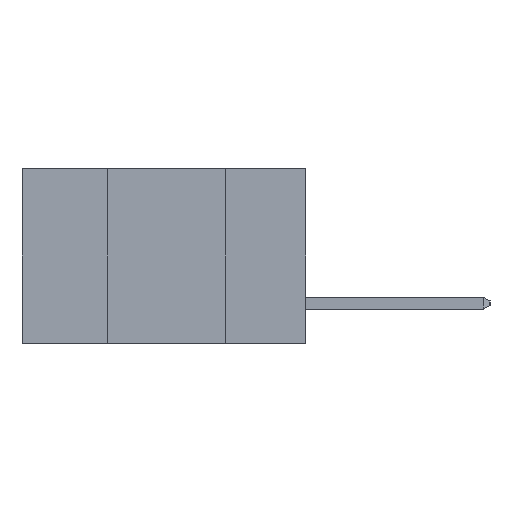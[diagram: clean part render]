
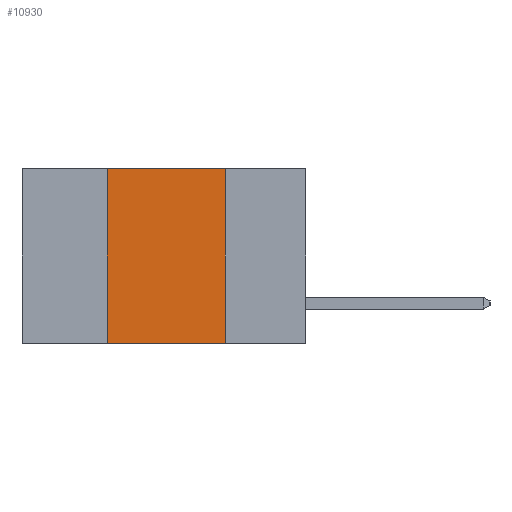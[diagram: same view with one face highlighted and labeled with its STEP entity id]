
A CAD part, left-side view. The second image highlights one B-rep face of the part: STEP entity #10930.
In plain terms, the highlighted planar face has unit normal (-1, 0, 0).
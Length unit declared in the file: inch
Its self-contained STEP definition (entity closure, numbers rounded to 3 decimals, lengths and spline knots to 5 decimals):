
#370 = VERTEX_POINT ( 'NONE', #13220 ) ;
#818 = VECTOR ( 'NONE', #9403, 39.37008 ) ;
#1462 = EDGE_CURVE ( 'NONE', #370, #1573, #7725, .T. ) ;
#1573 = VERTEX_POINT ( 'NONE', #4382 ) ;
#2150 = VECTOR ( 'NONE', #5373, 39.37008 ) ;
#2294 = EDGE_CURVE ( 'NONE', #1573, #11565, #12424, .T. ) ;
#3487 = VECTOR ( 'NONE', #15540, 39.37008 ) ;
#3701 = DIRECTION ( 'NONE',  ( 1., 0., 0. ) ) ;
#3955 = CARTESIAN_POINT ( 'NONE',  ( 0., 0.17, -0.37 ) ) ;
#4382 = CARTESIAN_POINT ( 'NONE',  ( 0., 0.17, 0. ) ) ;
#5013 = EDGE_CURVE ( 'NONE', #12340, #11565, #13702, .T. ) ;
#5373 = DIRECTION ( 'NONE',  ( 0., 0., -1. ) ) ;
#5451 = FACE_OUTER_BOUND ( 'NONE', #8555, .T. ) ;
#5587 = ORIENTED_EDGE ( 'NONE', *, *, #1462, .F. ) ;
#6796 = CARTESIAN_POINT ( 'NONE',  ( 0., 0.42, 0. ) ) ;
#7725 = LINE ( 'NONE', #14478, #818 ) ;
#8081 = DIRECTION ( 'NONE',  ( 0., 0., 1. ) ) ;
#8555 = EDGE_LOOP ( 'NONE', ( #11307, #5587, #14838, #9455 ) ) ;
#8854 = PLANE ( 'NONE',  #11930 ) ;
#9403 = DIRECTION ( 'NONE',  ( 0., -1., 0. ) ) ;
#9455 = ORIENTED_EDGE ( 'NONE', *, *, #5013, .T. ) ;
#10692 = VECTOR ( 'NONE', #8081, 39.37008 ) ;
#10930 = ADVANCED_FACE ( 'NONE', ( #5451 ), #8854, .F. ) ;
#11307 = ORIENTED_EDGE ( 'NONE', *, *, #2294, .F. ) ;
#11390 = CARTESIAN_POINT ( 'NONE',  ( 0., 0.6, 0. ) ) ;
#11565 = VERTEX_POINT ( 'NONE', #3955 ) ;
#11594 = CARTESIAN_POINT ( 'NONE',  ( 0., 0.17, 0. ) ) ;
#11930 = AXIS2_PLACEMENT_3D ( 'NONE', #11390, #3701, #12666 ) ;
#12202 = CARTESIAN_POINT ( 'NONE',  ( 0., 0.42, -0.37 ) ) ;
#12340 = VERTEX_POINT ( 'NONE', #12202 ) ;
#12424 = LINE ( 'NONE', #11594, #2150 ) ;
#12666 = DIRECTION ( 'NONE',  ( 0., 0., -1. ) ) ;
#12839 = CARTESIAN_POINT ( 'NONE',  ( 0., 0.6, -0.37 ) ) ;
#13220 = CARTESIAN_POINT ( 'NONE',  ( 0., 0.42, 0. ) ) ;
#13702 = LINE ( 'NONE', #12839, #3487 ) ;
#13786 = EDGE_CURVE ( 'NONE', #12340, #370, #14127, .T. ) ;
#14127 = LINE ( 'NONE', #6796, #10692 ) ;
#14478 = CARTESIAN_POINT ( 'NONE',  ( 0., 0.6, 0. ) ) ;
#14838 = ORIENTED_EDGE ( 'NONE', *, *, #13786, .F. ) ;
#15540 = DIRECTION ( 'NONE',  ( 0., -1., 0. ) ) ;
